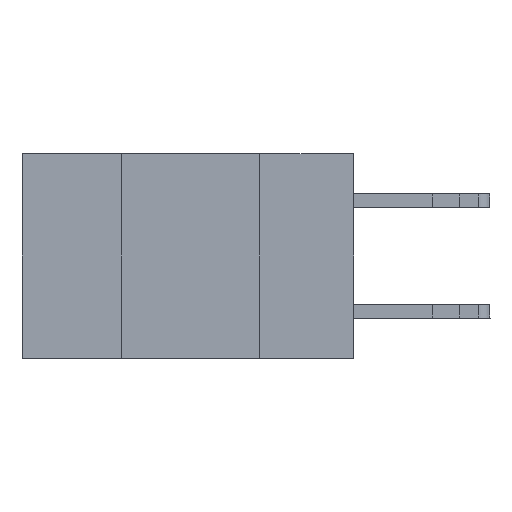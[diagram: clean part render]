
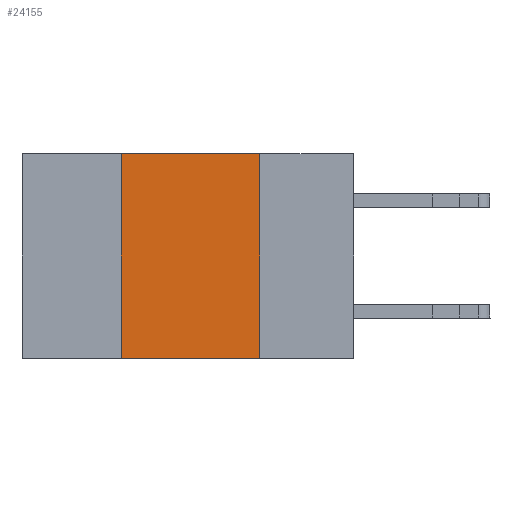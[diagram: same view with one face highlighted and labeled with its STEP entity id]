
A CAD part, left-side view. The second image highlights one B-rep face of the part: STEP entity #24155.
In plain terms, the highlighted planar face has unit normal (-1, 0, 0).
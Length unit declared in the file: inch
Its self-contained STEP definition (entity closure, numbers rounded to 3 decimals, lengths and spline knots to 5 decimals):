
#432 = CARTESIAN_POINT ( 'NONE',  ( 0., 0.42, -0.37 ) ) ;
#1175 = FACE_OUTER_BOUND ( 'NONE', #20464, .T. ) ;
#3069 = DIRECTION ( 'NONE',  ( 0., 0., 1. ) ) ;
#3304 = EDGE_CURVE ( 'NONE', #9996, #18547, #3817, .T. ) ;
#3624 = PLANE ( 'NONE',  #9439 ) ;
#3817 = LINE ( 'NONE', #29507, #18972 ) ;
#4107 = VECTOR ( 'NONE', #6894, 39.37008 ) ;
#4579 = EDGE_CURVE ( 'NONE', #23997, #9996, #26316, .T. ) ;
#6724 = ORIENTED_EDGE ( 'NONE', *, *, #7065, .F. ) ;
#6837 = CARTESIAN_POINT ( 'NONE',  ( 0., 0.17, 0. ) ) ;
#6894 = DIRECTION ( 'NONE',  ( 0., -1., 0. ) ) ;
#6905 = CARTESIAN_POINT ( 'NONE',  ( 0., 0.17, -0.37 ) ) ;
#7065 = EDGE_CURVE ( 'NONE', #18547, #21026, #11580, .T. ) ;
#9439 = AXIS2_PLACEMENT_3D ( 'NONE', #15092, #20285, #29318 ) ;
#9488 = CARTESIAN_POINT ( 'NONE',  ( 0., 0.6, -0.37 ) ) ;
#9996 = VERTEX_POINT ( 'NONE', #26467 ) ;
#10730 = VECTOR ( 'NONE', #3069, 39.37008 ) ;
#11580 = LINE ( 'NONE', #6837, #18078 ) ;
#12060 = ORIENTED_EDGE ( 'NONE', *, *, #4579, .F. ) ;
#13575 = DIRECTION ( 'NONE',  ( 0., 0., -1. ) ) ;
#15092 = CARTESIAN_POINT ( 'NONE',  ( 0., 0.6, 0. ) ) ;
#16578 = ORIENTED_EDGE ( 'NONE', *, *, #26650, .T. ) ;
#17877 = ORIENTED_EDGE ( 'NONE', *, *, #3304, .F. ) ;
#18078 = VECTOR ( 'NONE', #13575, 39.37008 ) ;
#18547 = VERTEX_POINT ( 'NONE', #20589 ) ;
#18972 = VECTOR ( 'NONE', #20172, 39.37008 ) ;
#20172 = DIRECTION ( 'NONE',  ( 0., -1., 0. ) ) ;
#20285 = DIRECTION ( 'NONE',  ( 1., 0., 0. ) ) ;
#20464 = EDGE_LOOP ( 'NONE', ( #6724, #17877, #12060, #16578 ) ) ;
#20589 = CARTESIAN_POINT ( 'NONE',  ( 0., 0.17, 0. ) ) ;
#21026 = VERTEX_POINT ( 'NONE', #6905 ) ;
#23997 = VERTEX_POINT ( 'NONE', #432 ) ;
#24020 = CARTESIAN_POINT ( 'NONE',  ( 0., 0.42, 0. ) ) ;
#24155 = ADVANCED_FACE ( 'NONE', ( #1175 ), #3624, .F. ) ;
#25548 = LINE ( 'NONE', #9488, #4107 ) ;
#26316 = LINE ( 'NONE', #24020, #10730 ) ;
#26467 = CARTESIAN_POINT ( 'NONE',  ( 0., 0.42, 0. ) ) ;
#26650 = EDGE_CURVE ( 'NONE', #23997, #21026, #25548, .T. ) ;
#29318 = DIRECTION ( 'NONE',  ( 0., 0., -1. ) ) ;
#29507 = CARTESIAN_POINT ( 'NONE',  ( 0., 0.6, 0. ) ) ;
